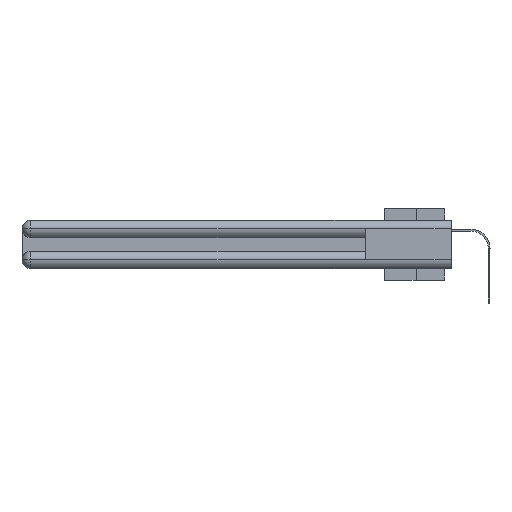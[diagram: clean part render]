
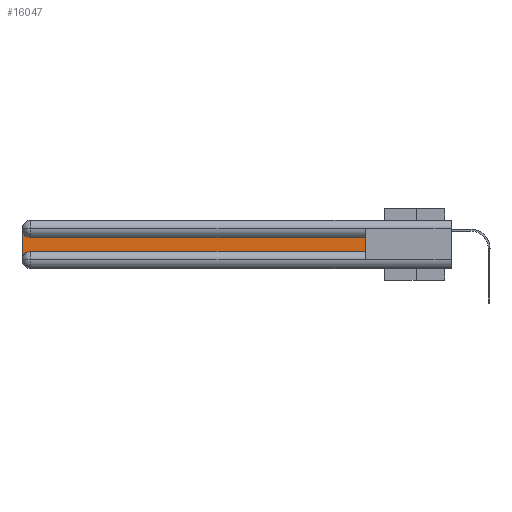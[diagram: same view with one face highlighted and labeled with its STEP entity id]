
A CAD part, left-side view. The second image highlights one B-rep face of the part: STEP entity #16047.
In plain terms, the highlighted planar face has unit normal (-1, 0, 0).
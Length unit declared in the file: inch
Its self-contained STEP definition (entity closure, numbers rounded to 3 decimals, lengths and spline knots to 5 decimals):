
#1555 = VECTOR ( 'NONE', #12847, 39.37008 ) ;
#2048 = VERTEX_POINT ( 'NONE', #33970 ) ;
#4140 = FACE_OUTER_BOUND ( 'NONE', #8450, .T. ) ;
#4463 = ORIENTED_EDGE ( 'NONE', *, *, #35743, .T. ) ;
#5735 = AXIS2_PLACEMENT_3D ( 'NONE', #31047, #30865, #31578 ) ;
#5782 = ORIENTED_EDGE ( 'NONE', *, *, #11633, .T. ) ;
#6485 = CARTESIAN_POINT ( 'NONE',  ( 0.075, 2.94, -0.0625 ) ) ;
#6646 = DIRECTION ( 'NONE',  ( 0., 0., -1. ) ) ;
#6884 = AXIS2_PLACEMENT_3D ( 'NONE', #15391, #27047, #30003 ) ;
#7972 = VERTEX_POINT ( 'NONE', #8058 ) ;
#7992 = CARTESIAN_POINT ( 'NONE',  ( 0.075, 0.6, -0.2175 ) ) ;
#8058 = CARTESIAN_POINT ( 'NONE',  ( 0.075, 2.94, -0.2175 ) ) ;
#8450 = EDGE_LOOP ( 'NONE', ( #30021, #5782, #22527, #4463, #24851, #32946 ) ) ;
#9585 = CARTESIAN_POINT ( 'NONE',  ( 0.075, 0.6, -0.1225 ) ) ;
#9589 = DIRECTION ( 'NONE',  ( 0., 0., -1. ) ) ;
#10416 = EDGE_CURVE ( 'NONE', #2048, #14733, #12370, .T. ) ;
#11633 = EDGE_CURVE ( 'NONE', #12706, #2048, #35145, .T. ) ;
#12370 = LINE ( 'NONE', #20686, #22509 ) ;
#12706 = VERTEX_POINT ( 'NONE', #23227 ) ;
#12847 = DIRECTION ( 'NONE',  ( 0., 0., 1. ) ) ;
#14733 = VERTEX_POINT ( 'NONE', #16155 ) ;
#15146 = EDGE_CURVE ( 'NONE', #7972, #25020, #24429, .T. ) ;
#15391 = CARTESIAN_POINT ( 'NONE',  ( 0.075, 3., -0.1225 ) ) ;
#15761 = PLANE ( 'NONE',  #6884 ) ;
#16047 = ADVANCED_FACE ( 'NONE', ( #4140 ), #15761, .F. ) ;
#16155 = CARTESIAN_POINT ( 'NONE',  ( 0.075, 3., -0.2775 ) ) ;
#16292 = DIRECTION ( 'NONE',  ( 0., -1., 0. ) ) ;
#17734 = LINE ( 'NONE', #9585, #34591 ) ;
#18559 = LINE ( 'NONE', #18945, #1555 ) ;
#18945 = CARTESIAN_POINT ( 'NONE',  ( 0.075, 0.6, -0.2175 ) ) ;
#19824 = AXIS2_PLACEMENT_3D ( 'NONE', #6485, #20861, #9589 ) ;
#20686 = CARTESIAN_POINT ( 'NONE',  ( 0.075, 3., -0.2175 ) ) ;
#20857 = DIRECTION ( 'NONE',  ( 0., 1., 0. ) ) ;
#20861 = DIRECTION ( 'NONE',  ( 1., 0., 0. ) ) ;
#21269 = EDGE_CURVE ( 'NONE', #21858, #12706, #17734, .T. ) ;
#21858 = VERTEX_POINT ( 'NONE', #26919 ) ;
#22509 = VECTOR ( 'NONE', #6646, 39.37008 ) ;
#22527 = ORIENTED_EDGE ( 'NONE', *, *, #10416, .T. ) ;
#23227 = CARTESIAN_POINT ( 'NONE',  ( 0.075, 2.94, -0.1225 ) ) ;
#24429 = LINE ( 'NONE', #7992, #24522 ) ;
#24522 = VECTOR ( 'NONE', #16292, 39.37008 ) ;
#24851 = ORIENTED_EDGE ( 'NONE', *, *, #15146, .T. ) ;
#25020 = VERTEX_POINT ( 'NONE', #33619 ) ;
#26919 = CARTESIAN_POINT ( 'NONE',  ( 0.075, 0.6, -0.1225 ) ) ;
#27047 = DIRECTION ( 'NONE',  ( 1., 0., 0. ) ) ;
#28760 = CIRCLE ( 'NONE', #5735, 0.06 ) ;
#30003 = DIRECTION ( 'NONE',  ( 0., 0., -1. ) ) ;
#30021 = ORIENTED_EDGE ( 'NONE', *, *, #21269, .T. ) ;
#30865 = DIRECTION ( 'NONE',  ( 1., 0., 0. ) ) ;
#31047 = CARTESIAN_POINT ( 'NONE',  ( 0.075, 2.94, -0.2775 ) ) ;
#31578 = DIRECTION ( 'NONE',  ( 0., 0., -1. ) ) ;
#32946 = ORIENTED_EDGE ( 'NONE', *, *, #35170, .T. ) ;
#33619 = CARTESIAN_POINT ( 'NONE',  ( 0.075, 0.6, -0.2175 ) ) ;
#33970 = CARTESIAN_POINT ( 'NONE',  ( 0.075, 3., -0.0625 ) ) ;
#34591 = VECTOR ( 'NONE', #20857, 39.37008 ) ;
#35145 = CIRCLE ( 'NONE', #19824, 0.06 ) ;
#35170 = EDGE_CURVE ( 'NONE', #25020, #21858, #18559, .T. ) ;
#35743 = EDGE_CURVE ( 'NONE', #14733, #7972, #28760, .T. ) ;
